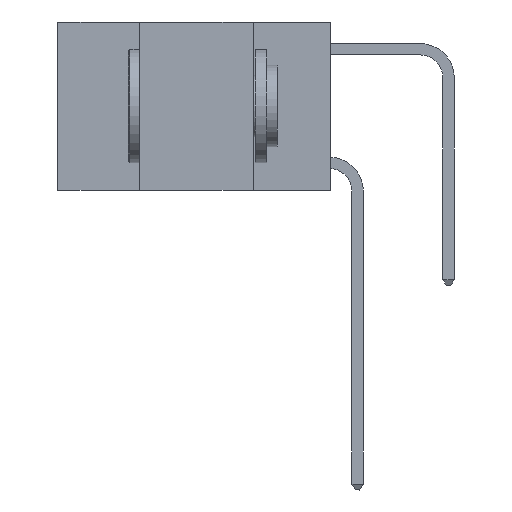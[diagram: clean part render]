
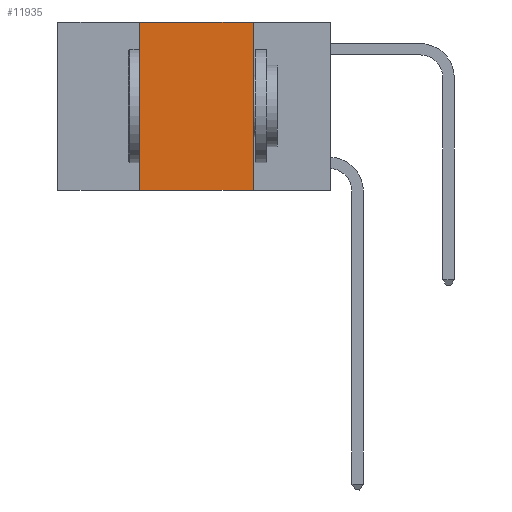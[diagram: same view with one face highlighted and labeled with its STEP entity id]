
A CAD part, left-side view. The second image highlights one B-rep face of the part: STEP entity #11935.
In plain terms, the highlighted planar face has unit normal (-1, 0, 0).
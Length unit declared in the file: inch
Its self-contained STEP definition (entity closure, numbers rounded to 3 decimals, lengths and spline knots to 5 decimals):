
#1093 = DIRECTION ( 'NONE',  ( 0., 0., 1. ) ) ;
#1131 = CARTESIAN_POINT ( 'NONE',  ( 0., 0.42, 0. ) ) ;
#1586 = VERTEX_POINT ( 'NONE', #6693 ) ;
#1710 = VECTOR ( 'NONE', #1093, 39.37008 ) ;
#1859 = VERTEX_POINT ( 'NONE', #9848 ) ;
#2394 = PLANE ( 'NONE',  #9463 ) ;
#3112 = FACE_OUTER_BOUND ( 'NONE', #11584, .T. ) ;
#3396 = LINE ( 'NONE', #8735, #6958 ) ;
#3917 = DIRECTION ( 'NONE',  ( 0., -1., 0. ) ) ;
#3981 = EDGE_CURVE ( 'NONE', #1859, #1586, #5086, .T. ) ;
#4039 = CARTESIAN_POINT ( 'NONE',  ( 0., 0.6, -0.37 ) ) ;
#4396 = CARTESIAN_POINT ( 'NONE',  ( 0., 0.6, 0. ) ) ;
#4841 = ORIENTED_EDGE ( 'NONE', *, *, #3981, .T. ) ;
#4906 = EDGE_CURVE ( 'NONE', #6062, #9955, #3396, .T. ) ;
#4947 = DIRECTION ( 'NONE',  ( 0., -1., 0. ) ) ;
#5021 = LINE ( 'NONE', #9599, #5172 ) ;
#5086 = LINE ( 'NONE', #4039, #9976 ) ;
#5172 = VECTOR ( 'NONE', #11678, 39.37008 ) ;
#6062 = VERTEX_POINT ( 'NONE', #11405 ) ;
#6693 = CARTESIAN_POINT ( 'NONE',  ( 0., 0.17, -0.37 ) ) ;
#6958 = VECTOR ( 'NONE', #4947, 39.37008 ) ;
#7212 = ORIENTED_EDGE ( 'NONE', *, *, #9674, .F. ) ;
#8026 = CARTESIAN_POINT ( 'NONE',  ( 0., 0.17, 0. ) ) ;
#8167 = DIRECTION ( 'NONE',  ( 0., 0., -1. ) ) ;
#8735 = CARTESIAN_POINT ( 'NONE',  ( 0., 0.6, 0. ) ) ;
#9329 = LINE ( 'NONE', #1131, #1710 ) ;
#9463 = AXIS2_PLACEMENT_3D ( 'NONE', #4396, #12148, #8167 ) ;
#9599 = CARTESIAN_POINT ( 'NONE',  ( 0., 0.17, 0. ) ) ;
#9674 = EDGE_CURVE ( 'NONE', #9955, #1586, #5021, .T. ) ;
#9727 = ORIENTED_EDGE ( 'NONE', *, *, #4906, .F. ) ;
#9737 = EDGE_CURVE ( 'NONE', #1859, #6062, #9329, .T. ) ;
#9848 = CARTESIAN_POINT ( 'NONE',  ( 0., 0.42, -0.37 ) ) ;
#9955 = VERTEX_POINT ( 'NONE', #8026 ) ;
#9976 = VECTOR ( 'NONE', #3917, 39.37008 ) ;
#11405 = CARTESIAN_POINT ( 'NONE',  ( 0., 0.42, 0. ) ) ;
#11584 = EDGE_LOOP ( 'NONE', ( #7212, #9727, #12137, #4841 ) ) ;
#11678 = DIRECTION ( 'NONE',  ( 0., 0., -1. ) ) ;
#11935 = ADVANCED_FACE ( 'NONE', ( #3112 ), #2394, .F. ) ;
#12137 = ORIENTED_EDGE ( 'NONE', *, *, #9737, .F. ) ;
#12148 = DIRECTION ( 'NONE',  ( 1., 0., 0. ) ) ;
